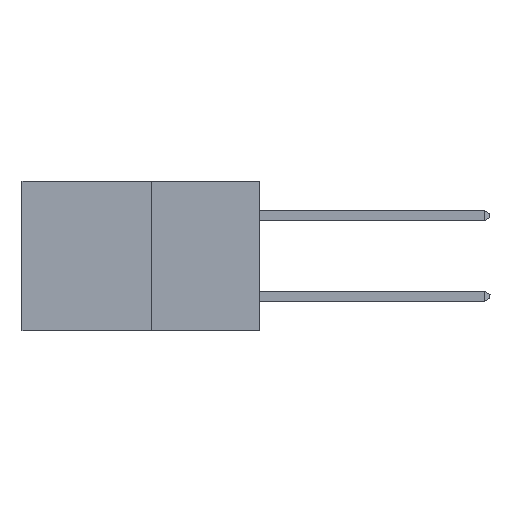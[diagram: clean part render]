
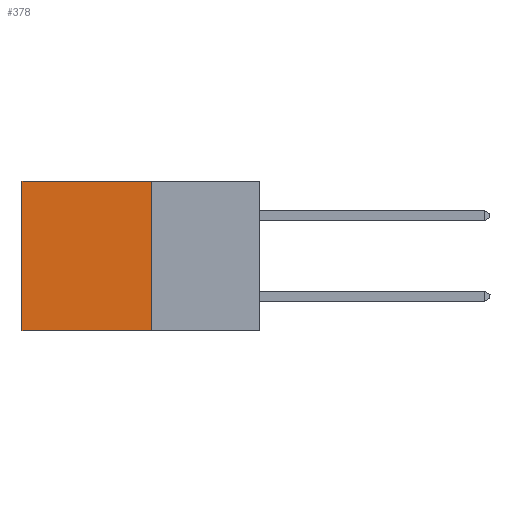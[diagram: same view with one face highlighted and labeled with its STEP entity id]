
A CAD part, left-side view. The second image highlights one B-rep face of the part: STEP entity #378.
In plain terms, the highlighted planar face has unit normal (-1, 0, 0).
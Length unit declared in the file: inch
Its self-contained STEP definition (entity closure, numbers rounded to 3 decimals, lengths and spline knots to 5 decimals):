
#80 = LINE ( 'NONE', #1961, #5295 ) ;
#110 = FACE_OUTER_BOUND ( 'NONE', #334, .T. ) ;
#126 = CARTESIAN_POINT ( 'NONE',  ( 0.277, 0.59, -0.37 ) ) ;
#334 = EDGE_LOOP ( 'NONE', ( #1007, #6181, #7475, #3563 ) ) ;
#378 = ADVANCED_FACE ( 'NONE', ( #110 ), #1267, .F. ) ;
#385 = DIRECTION ( 'NONE',  ( 0., 1., 0. ) ) ;
#1004 = DIRECTION ( 'NONE',  ( 0., 0., -1. ) ) ;
#1007 = ORIENTED_EDGE ( 'NONE', *, *, #4810, .T. ) ;
#1267 = PLANE ( 'NONE',  #2956 ) ;
#1532 = EDGE_CURVE ( 'NONE', #3220, #6387, #5421, .T. ) ;
#1799 = DIRECTION ( 'NONE',  ( 0., 1., 0. ) ) ;
#1848 = LINE ( 'NONE', #1937, #7869 ) ;
#1937 = CARTESIAN_POINT ( 'NONE',  ( 0.277, 0.27, -0.37 ) ) ;
#1961 = CARTESIAN_POINT ( 'NONE',  ( 0.277, 0.27, 0. ) ) ;
#2956 = AXIS2_PLACEMENT_3D ( 'NONE', #5488, #7576, #4921 ) ;
#3220 = VERTEX_POINT ( 'NONE', #3796 ) ;
#3563 = ORIENTED_EDGE ( 'NONE', *, *, #4459, .T. ) ;
#3796 = CARTESIAN_POINT ( 'NONE',  ( 0.277, 0.27, 0. ) ) ;
#4459 = EDGE_CURVE ( 'NONE', #3220, #7467, #80, .T. ) ;
#4476 = CARTESIAN_POINT ( 'NONE',  ( 0.277, 0.59, -0.37 ) ) ;
#4653 = LINE ( 'NONE', #126, #7266 ) ;
#4793 = CARTESIAN_POINT ( 'NONE',  ( 0.277, 0.27, -0.37 ) ) ;
#4810 = EDGE_CURVE ( 'NONE', #7467, #5927, #4653, .T. ) ;
#4893 = CARTESIAN_POINT ( 'NONE',  ( 0.277, 0.59, 0. ) ) ;
#4921 = DIRECTION ( 'NONE',  ( 0., 0., -1. ) ) ;
#5242 = VECTOR ( 'NONE', #6740, 39.37008 ) ;
#5295 = VECTOR ( 'NONE', #1799, 39.37008 ) ;
#5421 = LINE ( 'NONE', #4793, #5242 ) ;
#5488 = CARTESIAN_POINT ( 'NONE',  ( 0.277, 0.27, -0.37 ) ) ;
#5927 = VERTEX_POINT ( 'NONE', #4476 ) ;
#6181 = ORIENTED_EDGE ( 'NONE', *, *, #6457, .F. ) ;
#6387 = VERTEX_POINT ( 'NONE', #7274 ) ;
#6457 = EDGE_CURVE ( 'NONE', #6387, #5927, #1848, .T. ) ;
#6740 = DIRECTION ( 'NONE',  ( 0., 0., -1. ) ) ;
#7266 = VECTOR ( 'NONE', #1004, 39.37008 ) ;
#7274 = CARTESIAN_POINT ( 'NONE',  ( 0.277, 0.27, -0.37 ) ) ;
#7467 = VERTEX_POINT ( 'NONE', #4893 ) ;
#7475 = ORIENTED_EDGE ( 'NONE', *, *, #1532, .F. ) ;
#7576 = DIRECTION ( 'NONE',  ( 1., 0., 0. ) ) ;
#7869 = VECTOR ( 'NONE', #385, 39.37008 ) ;
